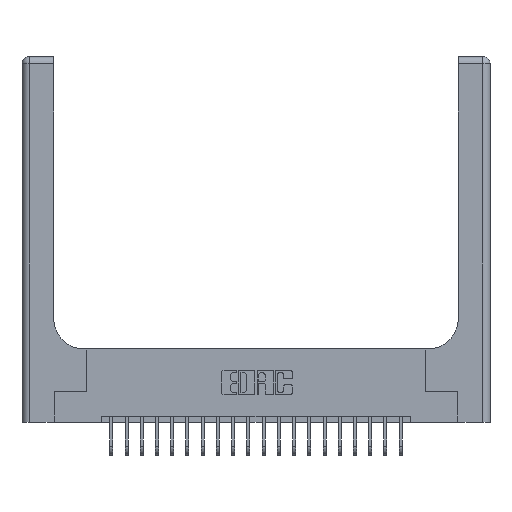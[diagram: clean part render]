
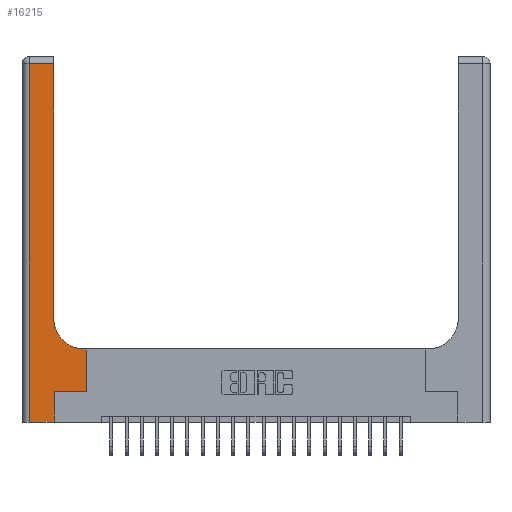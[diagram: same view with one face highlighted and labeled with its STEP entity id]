
A CAD part, top view. The second image highlights one B-rep face of the part: STEP entity #16215.
In plain terms, the highlighted planar face has unit normal (0, 0, 1).
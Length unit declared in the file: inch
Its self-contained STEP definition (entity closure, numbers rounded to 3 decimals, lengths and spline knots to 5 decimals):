
#100 = ORIENTED_EDGE ( 'NONE', *, *, #1060, .T. ) ;
#102 = EDGE_CURVE ( 'NONE', #22874, #5686, #4407, .T. ) ;
#1002 = AXIS2_PLACEMENT_3D ( 'NONE', #17831, #3649, #19733 ) ;
#1059 = CARTESIAN_POINT ( 'NONE',  ( 0.528, 0.6, 0.37 ) ) ;
#1060 = EDGE_CURVE ( 'NONE', #22638, #13048, #14969, .T. ) ;
#1147 = VERTEX_POINT ( 'NONE', #11341 ) ;
#1974 = EDGE_LOOP ( 'NONE', ( #3498, #21931, #10773, #10249, #100, #1981, #4441, #22337, #9701 ) ) ;
#1981 = ORIENTED_EDGE ( 'NONE', *, *, #10808, .T. ) ;
#2125 = VECTOR ( 'NONE', #18552, 39.37008 ) ;
#2264 = DIRECTION ( 'NONE',  ( 0., 0., -1. ) ) ;
#2327 = EDGE_CURVE ( 'NONE', #8460, #12980, #7971, .T. ) ;
#3372 = DIRECTION ( 'NONE',  ( -1., 0., 0. ) ) ;
#3498 = ORIENTED_EDGE ( 'NONE', *, *, #3591, .T. ) ;
#3591 = EDGE_CURVE ( 'NONE', #5686, #1147, #9090, .T. ) ;
#3649 = DIRECTION ( 'NONE',  ( 0., 0., -1. ) ) ;
#4282 = LINE ( 'NONE', #18238, #20967 ) ;
#4407 = CIRCLE ( 'NONE', #1002, 0.25 ) ;
#4441 = ORIENTED_EDGE ( 'NONE', *, *, #11768, .T. ) ;
#4468 = DIRECTION ( 'NONE',  ( 1., 0., 0. ) ) ;
#5671 = VERTEX_POINT ( 'NONE', #17719 ) ;
#5686 = VERTEX_POINT ( 'NONE', #14030 ) ;
#5790 = CARTESIAN_POINT ( 'NONE',  ( 0.06, 0., 0.37 ) ) ;
#5941 = EDGE_CURVE ( 'NONE', #12980, #22638, #4282, .T. ) ;
#6082 = VERTEX_POINT ( 'NONE', #1059 ) ;
#6092 = CARTESIAN_POINT ( 'NONE',  ( 0.26, 3., 0.37 ) ) ;
#6193 = AXIS2_PLACEMENT_3D ( 'NONE', #21616, #2264, #14481 ) ;
#6378 = VECTOR ( 'NONE', #15949, 39.37008 ) ;
#6846 = CARTESIAN_POINT ( 'NONE',  ( 0.265, 0.25, 0.37 ) ) ;
#6881 = EDGE_CURVE ( 'NONE', #1147, #8460, #13200, .T. ) ;
#7400 = CARTESIAN_POINT ( 'NONE',  ( 0.265, 0., 0.37 ) ) ;
#7971 = LINE ( 'NONE', #19567, #13769 ) ;
#8460 = VERTEX_POINT ( 'NONE', #19044 ) ;
#8654 = EDGE_CURVE ( 'NONE', #6082, #22874, #13731, .T. ) ;
#9090 = LINE ( 'NONE', #6092, #2125 ) ;
#9187 = PLANE ( 'NONE',  #6193 ) ;
#9701 = ORIENTED_EDGE ( 'NONE', *, *, #102, .T. ) ;
#10249 = ORIENTED_EDGE ( 'NONE', *, *, #5941, .T. ) ;
#10715 = DIRECTION ( 'NONE',  ( 0., 1., 0. ) ) ;
#10773 = ORIENTED_EDGE ( 'NONE', *, *, #2327, .T. ) ;
#10808 = EDGE_CURVE ( 'NONE', #13048, #5671, #17269, .T. ) ;
#11341 = CARTESIAN_POINT ( 'NONE',  ( 0.26, 2.94, 0.37 ) ) ;
#11768 = EDGE_CURVE ( 'NONE', #5671, #6082, #14239, .T. ) ;
#12594 = DIRECTION ( 'NONE',  ( 0., -1., 0. ) ) ;
#12980 = VERTEX_POINT ( 'NONE', #5790 ) ;
#13048 = VERTEX_POINT ( 'NONE', #18648 ) ;
#13200 = LINE ( 'NONE', #21322, #13753 ) ;
#13731 = LINE ( 'NONE', #19492, #19035 ) ;
#13753 = VECTOR ( 'NONE', #3372, 39.37008 ) ;
#13769 = VECTOR ( 'NONE', #12594, 39.37008 ) ;
#14030 = CARTESIAN_POINT ( 'NONE',  ( 0.26, 0.85, 0.37 ) ) ;
#14239 = LINE ( 'NONE', #15256, #14790 ) ;
#14481 = DIRECTION ( 'NONE',  ( -1., 0., 0. ) ) ;
#14790 = VECTOR ( 'NONE', #17060, 39.37008 ) ;
#14969 = LINE ( 'NONE', #17757, #22162 ) ;
#15256 = CARTESIAN_POINT ( 'NONE',  ( 0.528, 0.25, 0.37 ) ) ;
#15949 = DIRECTION ( 'NONE',  ( 1., 0., 0. ) ) ;
#16215 = ADVANCED_FACE ( 'NONE', ( #20428 ), #9187, .F. ) ;
#17060 = DIRECTION ( 'NONE',  ( 0., 1., 0. ) ) ;
#17269 = LINE ( 'NONE', #6846, #6378 ) ;
#17719 = CARTESIAN_POINT ( 'NONE',  ( 0.528, 0.25, 0.37 ) ) ;
#17757 = CARTESIAN_POINT ( 'NONE',  ( 0.265, 0., 0.37 ) ) ;
#17831 = CARTESIAN_POINT ( 'NONE',  ( 0.51, 0.85, 0.37 ) ) ;
#18238 = CARTESIAN_POINT ( 'NONE',  ( 0., 0., 0.37 ) ) ;
#18552 = DIRECTION ( 'NONE',  ( 0., 1., 0. ) ) ;
#18648 = CARTESIAN_POINT ( 'NONE',  ( 0.265, 0.25, 0.37 ) ) ;
#19035 = VECTOR ( 'NONE', #19556, 39.37008 ) ;
#19044 = CARTESIAN_POINT ( 'NONE',  ( 0.06, 2.94, 0.37 ) ) ;
#19492 = CARTESIAN_POINT ( 'NONE',  ( 0.26, 0.6, 0.37 ) ) ;
#19556 = DIRECTION ( 'NONE',  ( -1., 0., 0. ) ) ;
#19567 = CARTESIAN_POINT ( 'NONE',  ( 0.06, 3., 0.37 ) ) ;
#19733 = DIRECTION ( 'NONE',  ( 1., 0., 0. ) ) ;
#20428 = FACE_OUTER_BOUND ( 'NONE', #1974, .T. ) ;
#20967 = VECTOR ( 'NONE', #4468, 39.37008 ) ;
#21322 = CARTESIAN_POINT ( 'NONE',  ( 0., 2.94, 0.37 ) ) ;
#21616 = CARTESIAN_POINT ( 'NONE',  ( 0., 3., 0.37 ) ) ;
#21931 = ORIENTED_EDGE ( 'NONE', *, *, #6881, .T. ) ;
#22162 = VECTOR ( 'NONE', #10715, 39.37008 ) ;
#22337 = ORIENTED_EDGE ( 'NONE', *, *, #8654, .T. ) ;
#22452 = CARTESIAN_POINT ( 'NONE',  ( 0.51, 0.6, 0.37 ) ) ;
#22638 = VERTEX_POINT ( 'NONE', #7400 ) ;
#22874 = VERTEX_POINT ( 'NONE', #22452 ) ;
